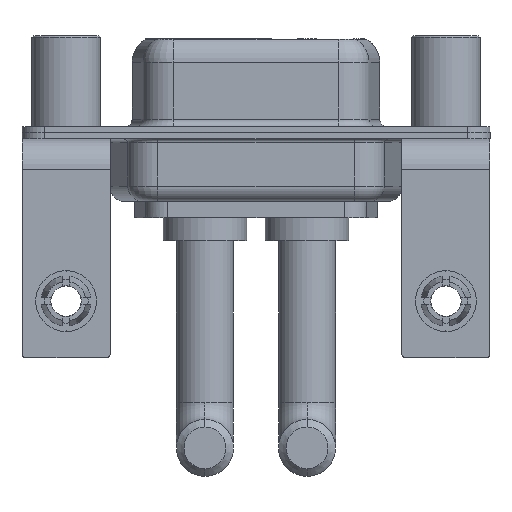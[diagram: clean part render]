
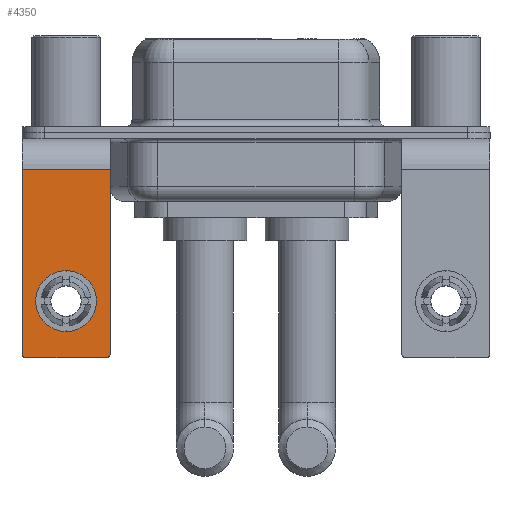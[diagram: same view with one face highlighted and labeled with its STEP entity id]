
A CAD part, front view. The second image highlights one B-rep face of the part: STEP entity #4350.
In plain terms, the highlighted planar face has unit normal (0, -1, 0).
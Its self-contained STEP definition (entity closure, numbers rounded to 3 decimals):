
#196 = VERTEX_POINT ( 'NONE', #5464 ) ;
#210 = DIRECTION ( 'NONE',  ( 0., 1., 0. ) ) ;
#252 = CARTESIAN_POINT ( 'NONE',  ( 2.9, -6.25, -2.4 ) ) ;
#712 = VERTEX_POINT ( 'NONE', #7991 ) ;
#716 = EDGE_CURVE ( 'NONE', #11461, #9546, #14303, .T. ) ;
#856 = DIRECTION ( 'NONE',  ( 0., -1., 0. ) ) ;
#1124 = AXIS2_PLACEMENT_3D ( 'NONE', #6273, #16670, #3566 ) ;
#1153 = CARTESIAN_POINT ( 'NONE',  ( -2.9, -6.25, -2.4 ) ) ;
#1846 = ORIENTED_EDGE ( 'NONE', *, *, #2767, .T. ) ;
#2032 = CARTESIAN_POINT ( 'NONE',  ( 2.9, -6.25, -2.4 ) ) ;
#2212 = VERTEX_POINT ( 'NONE', #8815 ) ;
#2265 = EDGE_CURVE ( 'NONE', #712, #10345, #7361, .T. ) ;
#2628 = DIRECTION ( 'NONE',  ( 0., 0., -1. ) ) ;
#2767 = EDGE_CURVE ( 'NONE', #712, #9546, #13024, .T. ) ;
#2854 = ORIENTED_EDGE ( 'NONE', *, *, #16319, .T. ) ;
#3431 = CARTESIAN_POINT ( 'NONE',  ( 2.65, -6.25, -14.55 ) ) ;
#3566 = DIRECTION ( 'NONE',  ( 0., 0., 1. ) ) ;
#4008 = EDGE_CURVE ( 'NONE', #6494, #10345, #13619, .T. ) ;
#4344 = DIRECTION ( 'NONE',  ( 0., 0., 1. ) ) ;
#4350 = ADVANCED_FACE ( 'NONE', ( #9391, #10995 ), #9471, .F. ) ;
#4408 = ORIENTED_EDGE ( 'NONE', *, *, #716, .F. ) ;
#4580 = ORIENTED_EDGE ( 'NONE', *, *, #15003, .T. ) ;
#4705 = DIRECTION ( 'NONE',  ( 0., -1., 0. ) ) ;
#4737 = CIRCLE ( 'NONE', #11535, 2. ) ;
#4800 = CARTESIAN_POINT ( 'NONE',  ( 0., -6.25, -9.07 ) ) ;
#4952 = CIRCLE ( 'NONE', #1124, 2. ) ;
#4993 = EDGE_CURVE ( 'NONE', #11461, #196, #10889, .T. ) ;
#5006 = LINE ( 'NONE', #1153, #16602 ) ;
#5464 = CARTESIAN_POINT ( 'NONE',  ( -2.9, -6.25, -2.4 ) ) ;
#5831 = ORIENTED_EDGE ( 'NONE', *, *, #9223, .T. ) ;
#6273 = CARTESIAN_POINT ( 'NONE',  ( 0., -6.25, -11.07 ) ) ;
#6494 = VERTEX_POINT ( 'NONE', #14190 ) ;
#6832 = VERTEX_POINT ( 'NONE', #4800 ) ;
#7242 = ORIENTED_EDGE ( 'NONE', *, *, #4993, .T. ) ;
#7361 = LINE ( 'NONE', #11277, #10898 ) ;
#7544 = CARTESIAN_POINT ( 'NONE',  ( 2.9, -6.25, -14.55 ) ) ;
#7991 = CARTESIAN_POINT ( 'NONE',  ( 2.65, -6.25, -14.8 ) ) ;
#8013 = CARTESIAN_POINT ( 'NONE',  ( 2.9, -6.25, -2.4 ) ) ;
#8063 = DIRECTION ( 'NONE',  ( 0., 0., 1. ) ) ;
#8619 = VECTOR ( 'NONE', #2628, 1000. ) ;
#8815 = CARTESIAN_POINT ( 'NONE',  ( 0., -6.25, -13.07 ) ) ;
#8982 = AXIS2_PLACEMENT_3D ( 'NONE', #11343, #856, #16377 ) ;
#9116 = EDGE_LOOP ( 'NONE', ( #5831, #2854 ) ) ;
#9223 = EDGE_CURVE ( 'NONE', #2212, #6832, #4737, .T. ) ;
#9253 = AXIS2_PLACEMENT_3D ( 'NONE', #8013, #13477, #4344 ) ;
#9391 = FACE_BOUND ( 'NONE', #9116, .T. ) ;
#9471 = PLANE ( 'NONE',  #9253 ) ;
#9546 = VERTEX_POINT ( 'NONE', #7544 ) ;
#9906 = DIRECTION ( 'NONE',  ( 0., 0., 1. ) ) ;
#9955 = DIRECTION ( 'NONE',  ( 0., 0., -1. ) ) ;
#10105 = VECTOR ( 'NONE', #13774, 1000. ) ;
#10345 = VERTEX_POINT ( 'NONE', #11146 ) ;
#10889 = LINE ( 'NONE', #2032, #10105 ) ;
#10898 = VECTOR ( 'NONE', #13668, 1000. ) ;
#10995 = FACE_OUTER_BOUND ( 'NONE', #12471, .T. ) ;
#11146 = CARTESIAN_POINT ( 'NONE',  ( -2.65, -6.25, -14.8 ) ) ;
#11277 = CARTESIAN_POINT ( 'NONE',  ( 2.9, -6.25, -14.8 ) ) ;
#11343 = CARTESIAN_POINT ( 'NONE',  ( -2.65, -6.25, -14.55 ) ) ;
#11393 = ORIENTED_EDGE ( 'NONE', *, *, #2265, .F. ) ;
#11461 = VERTEX_POINT ( 'NONE', #252 ) ;
#11535 = AXIS2_PLACEMENT_3D ( 'NONE', #11894, #210, #8063 ) ;
#11894 = CARTESIAN_POINT ( 'NONE',  ( 0., -6.25, -11.07 ) ) ;
#12471 = EDGE_LOOP ( 'NONE', ( #4580, #14881, #11393, #1846, #4408, #7242 ) ) ;
#12485 = AXIS2_PLACEMENT_3D ( 'NONE', #3431, #4705, #9906 ) ;
#13024 = CIRCLE ( 'NONE', #12485, 0.25 ) ;
#13477 = DIRECTION ( 'NONE',  ( 0., 1., 0. ) ) ;
#13619 = CIRCLE ( 'NONE', #8982, 0.25 ) ;
#13668 = DIRECTION ( 'NONE',  ( -1., 0., 0. ) ) ;
#13774 = DIRECTION ( 'NONE',  ( -1., 0., 0. ) ) ;
#14190 = CARTESIAN_POINT ( 'NONE',  ( -2.9, -6.25, -14.55 ) ) ;
#14303 = LINE ( 'NONE', #14566, #8619 ) ;
#14566 = CARTESIAN_POINT ( 'NONE',  ( 2.9, -6.25, -2.4 ) ) ;
#14881 = ORIENTED_EDGE ( 'NONE', *, *, #4008, .T. ) ;
#15003 = EDGE_CURVE ( 'NONE', #196, #6494, #5006, .T. ) ;
#16319 = EDGE_CURVE ( 'NONE', #6832, #2212, #4952, .T. ) ;
#16377 = DIRECTION ( 'NONE',  ( 0., 0., 1. ) ) ;
#16602 = VECTOR ( 'NONE', #9955, 1000. ) ;
#16670 = DIRECTION ( 'NONE',  ( 0., 1., 0. ) ) ;
